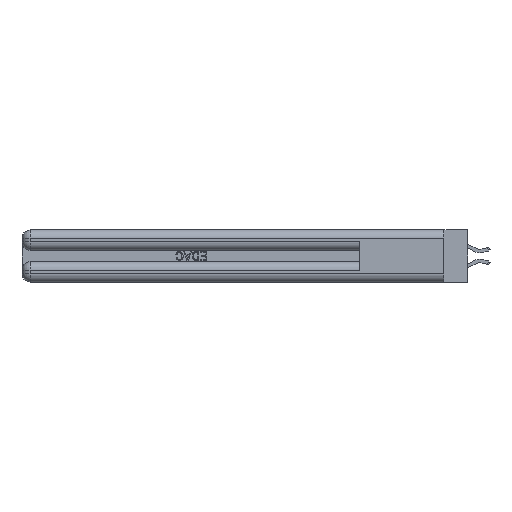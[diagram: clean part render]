
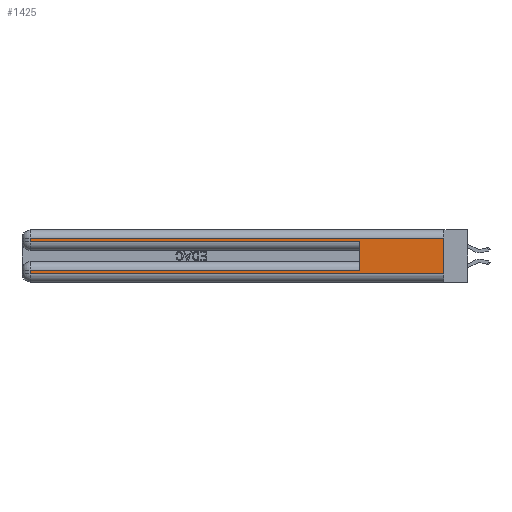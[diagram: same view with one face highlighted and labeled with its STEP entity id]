
A CAD part, left-side view. The second image highlights one B-rep face of the part: STEP entity #1425.
In plain terms, the highlighted planar face has unit normal (-1, 0, 0).
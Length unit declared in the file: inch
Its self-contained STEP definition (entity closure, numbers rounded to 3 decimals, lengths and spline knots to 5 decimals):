
#237 = CARTESIAN_POINT ( 'NONE',  ( 0., 0., 0.31 ) ) ;
#920 = VERTEX_POINT ( 'NONE', #35892 ) ;
#1425 = ADVANCED_FACE ( 'NONE', ( #30495 ), #28707, .F. ) ;
#4006 = LINE ( 'NONE', #40641, #35768 ) ;
#4566 = CARTESIAN_POINT ( 'NONE',  ( 0., 0., 0.37 ) ) ;
#4590 = LINE ( 'NONE', #14483, #20519 ) ;
#4657 = EDGE_CURVE ( 'NONE', #30592, #20918, #17395, .T. ) ;
#7162 = LINE ( 'NONE', #35154, #14589 ) ;
#7973 = VECTOR ( 'NONE', #18862, 39.37008 ) ;
#8157 = VECTOR ( 'NONE', #33045, 39.37008 ) ;
#8401 = VERTEX_POINT ( 'NONE', #33839 ) ;
#8886 = VECTOR ( 'NONE', #9829, 39.37008 ) ;
#9672 = CARTESIAN_POINT ( 'NONE',  ( 0., 0., 0.37 ) ) ;
#9829 = DIRECTION ( 'NONE',  ( 0., 0., 1. ) ) ;
#10668 = DIRECTION ( 'NONE',  ( 0., -1., 0. ) ) ;
#11208 = CARTESIAN_POINT ( 'NONE',  ( 0., 0., 0.06 ) ) ;
#12870 = DIRECTION ( 'NONE',  ( 0., 0., -1. ) ) ;
#14204 = ORIENTED_EDGE ( 'NONE', *, *, #34659, .T. ) ;
#14483 = CARTESIAN_POINT ( 'NONE',  ( 0., 0., 0.31 ) ) ;
#14517 = VERTEX_POINT ( 'NONE', #40510 ) ;
#14539 = EDGE_CURVE ( 'NONE', #25144, #21903, #4006, .T. ) ;
#14589 = VECTOR ( 'NONE', #19246, 39.37008 ) ;
#15203 = ORIENTED_EDGE ( 'NONE', *, *, #20760, .T. ) ;
#15223 = CARTESIAN_POINT ( 'NONE',  ( 0., 2.94, 0.37 ) ) ;
#15363 = DIRECTION ( 'NONE',  ( 0., 0., -1. ) ) ;
#17313 = LINE ( 'NONE', #22563, #8886 ) ;
#17381 = EDGE_CURVE ( 'NONE', #25144, #920, #17313, .T. ) ;
#17395 = LINE ( 'NONE', #37814, #7973 ) ;
#17667 = DIRECTION ( 'NONE',  ( 0., 1., 0. ) ) ;
#18862 = DIRECTION ( 'NONE',  ( 0., -1., 0. ) ) ;
#19246 = DIRECTION ( 'NONE',  ( 0., 0., -1. ) ) ;
#20519 = VECTOR ( 'NONE', #17667, 39.37008 ) ;
#20564 = LINE ( 'NONE', #15223, #37407 ) ;
#20760 = EDGE_CURVE ( 'NONE', #8401, #920, #37912, .T. ) ;
#20918 = VERTEX_POINT ( 'NONE', #11208 ) ;
#21164 = ORIENTED_EDGE ( 'NONE', *, *, #24410, .T. ) ;
#21903 = VERTEX_POINT ( 'NONE', #35360 ) ;
#22040 = VECTOR ( 'NONE', #10668, 39.37008 ) ;
#22563 = CARTESIAN_POINT ( 'NONE',  ( 0., 0.6, 0.145 ) ) ;
#22572 = EDGE_LOOP ( 'NONE', ( #37498, #14204, #39470, #15203, #33073, #36013, #21164, #38017 ) ) ;
#24237 = EDGE_CURVE ( 'NONE', #14517, #8401, #20564, .T. ) ;
#24410 = EDGE_CURVE ( 'NONE', #21903, #30592, #7162, .T. ) ;
#24888 = DIRECTION ( 'NONE',  ( 0., 1., 0. ) ) ;
#25144 = VERTEX_POINT ( 'NONE', #26416 ) ;
#26416 = CARTESIAN_POINT ( 'NONE',  ( 0., 0.6, 0.085 ) ) ;
#28707 = PLANE ( 'NONE',  #37152 ) ;
#29248 = CARTESIAN_POINT ( 'NONE',  ( 0., 2.94, 0.06 ) ) ;
#29683 = CARTESIAN_POINT ( 'NONE',  ( 0., 0., 0.285 ) ) ;
#30495 = FACE_OUTER_BOUND ( 'NONE', #22572, .T. ) ;
#30592 = VERTEX_POINT ( 'NONE', #29248 ) ;
#31745 = VERTEX_POINT ( 'NONE', #237 ) ;
#31868 = DIRECTION ( 'NONE',  ( 1., 0., 0. ) ) ;
#32465 = LINE ( 'NONE', #4566, #8157 ) ;
#33045 = DIRECTION ( 'NONE',  ( 0., 0., -1. ) ) ;
#33073 = ORIENTED_EDGE ( 'NONE', *, *, #17381, .F. ) ;
#33839 = CARTESIAN_POINT ( 'NONE',  ( 0., 2.94, 0.285 ) ) ;
#34371 = EDGE_CURVE ( 'NONE', #31745, #20918, #32465, .T. ) ;
#34659 = EDGE_CURVE ( 'NONE', #31745, #14517, #4590, .T. ) ;
#35154 = CARTESIAN_POINT ( 'NONE',  ( 0., 2.94, 0.37 ) ) ;
#35360 = CARTESIAN_POINT ( 'NONE',  ( 0., 2.94, 0.085 ) ) ;
#35768 = VECTOR ( 'NONE', #24888, 39.37008 ) ;
#35892 = CARTESIAN_POINT ( 'NONE',  ( 0., 0.6, 0.285 ) ) ;
#36013 = ORIENTED_EDGE ( 'NONE', *, *, #14539, .T. ) ;
#37152 = AXIS2_PLACEMENT_3D ( 'NONE', #9672, #31868, #12870 ) ;
#37407 = VECTOR ( 'NONE', #15363, 39.37008 ) ;
#37498 = ORIENTED_EDGE ( 'NONE', *, *, #34371, .F. ) ;
#37814 = CARTESIAN_POINT ( 'NONE',  ( 0., 0., 0.06 ) ) ;
#37912 = LINE ( 'NONE', #29683, #22040 ) ;
#38017 = ORIENTED_EDGE ( 'NONE', *, *, #4657, .T. ) ;
#39470 = ORIENTED_EDGE ( 'NONE', *, *, #24237, .T. ) ;
#40510 = CARTESIAN_POINT ( 'NONE',  ( 0., 2.94, 0.31 ) ) ;
#40641 = CARTESIAN_POINT ( 'NONE',  ( 0., 0., 0.085 ) ) ;
